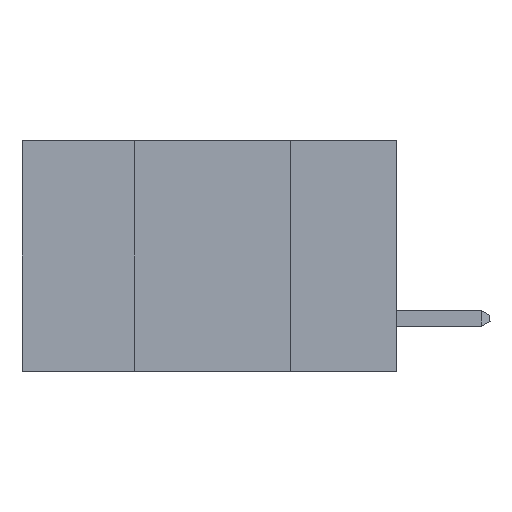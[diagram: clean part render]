
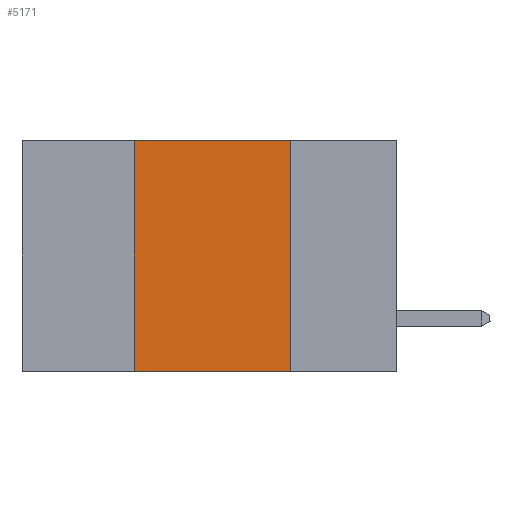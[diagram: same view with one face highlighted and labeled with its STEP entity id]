
A CAD part, left-side view. The second image highlights one B-rep face of the part: STEP entity #5171.
In plain terms, the highlighted planar face has unit normal (-1, 0, 0).
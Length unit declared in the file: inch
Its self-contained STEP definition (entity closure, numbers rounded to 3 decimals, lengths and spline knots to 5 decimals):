
#636 = CARTESIAN_POINT ( 'NONE',  ( 0., 0.6, -0.37 ) ) ;
#671 = FACE_OUTER_BOUND ( 'NONE', #2138, .T. ) ;
#690 = VECTOR ( 'NONE', #12045, 39.37008 ) ;
#1670 = VERTEX_POINT ( 'NONE', #10528 ) ;
#1737 = CARTESIAN_POINT ( 'NONE',  ( 0., 0.17, 0. ) ) ;
#1809 = PLANE ( 'NONE',  #11453 ) ;
#2105 = CARTESIAN_POINT ( 'NONE',  ( 0., 0.6, 0. ) ) ;
#2138 = EDGE_LOOP ( 'NONE', ( #8424, #11394, #11457, #9920 ) ) ;
#2690 = EDGE_CURVE ( 'NONE', #7258, #1670, #8346, .T. ) ;
#3081 = CARTESIAN_POINT ( 'NONE',  ( 0., 0.42, 0. ) ) ;
#3697 = LINE ( 'NONE', #2105, #12438 ) ;
#4345 = EDGE_CURVE ( 'NONE', #8016, #1670, #11241, .T. ) ;
#5171 = ADVANCED_FACE ( 'NONE', ( #671 ), #1809, .F. ) ;
#5196 = VERTEX_POINT ( 'NONE', #8702 ) ;
#5704 = DIRECTION ( 'NONE',  ( 0., 0., -1. ) ) ;
#5886 = DIRECTION ( 'NONE',  ( 0., 0., -1. ) ) ;
#6801 = VECTOR ( 'NONE', #8691, 39.37008 ) ;
#7148 = DIRECTION ( 'NONE',  ( 0., -1., 0. ) ) ;
#7258 = VERTEX_POINT ( 'NONE', #9522 ) ;
#7583 = EDGE_CURVE ( 'NONE', #5196, #8016, #3697, .T. ) ;
#8016 = VERTEX_POINT ( 'NONE', #11321 ) ;
#8346 = LINE ( 'NONE', #636, #6801 ) ;
#8424 = ORIENTED_EDGE ( 'NONE', *, *, #4345, .F. ) ;
#8619 = EDGE_CURVE ( 'NONE', #7258, #5196, #11935, .T. ) ;
#8691 = DIRECTION ( 'NONE',  ( 0., -1., 0. ) ) ;
#8702 = CARTESIAN_POINT ( 'NONE',  ( 0., 0.42, 0. ) ) ;
#9522 = CARTESIAN_POINT ( 'NONE',  ( 0., 0.42, -0.37 ) ) ;
#9695 = VECTOR ( 'NONE', #5704, 39.37008 ) ;
#9739 = DIRECTION ( 'NONE',  ( 1., 0., 0. ) ) ;
#9920 = ORIENTED_EDGE ( 'NONE', *, *, #2690, .T. ) ;
#10528 = CARTESIAN_POINT ( 'NONE',  ( 0., 0.17, -0.37 ) ) ;
#11241 = LINE ( 'NONE', #1737, #9695 ) ;
#11321 = CARTESIAN_POINT ( 'NONE',  ( 0., 0.17, 0. ) ) ;
#11394 = ORIENTED_EDGE ( 'NONE', *, *, #7583, .F. ) ;
#11453 = AXIS2_PLACEMENT_3D ( 'NONE', #11823, #9739, #5886 ) ;
#11457 = ORIENTED_EDGE ( 'NONE', *, *, #8619, .F. ) ;
#11823 = CARTESIAN_POINT ( 'NONE',  ( 0., 0.6, 0. ) ) ;
#11935 = LINE ( 'NONE', #3081, #690 ) ;
#12045 = DIRECTION ( 'NONE',  ( 0., 0., 1. ) ) ;
#12438 = VECTOR ( 'NONE', #7148, 39.37008 ) ;
